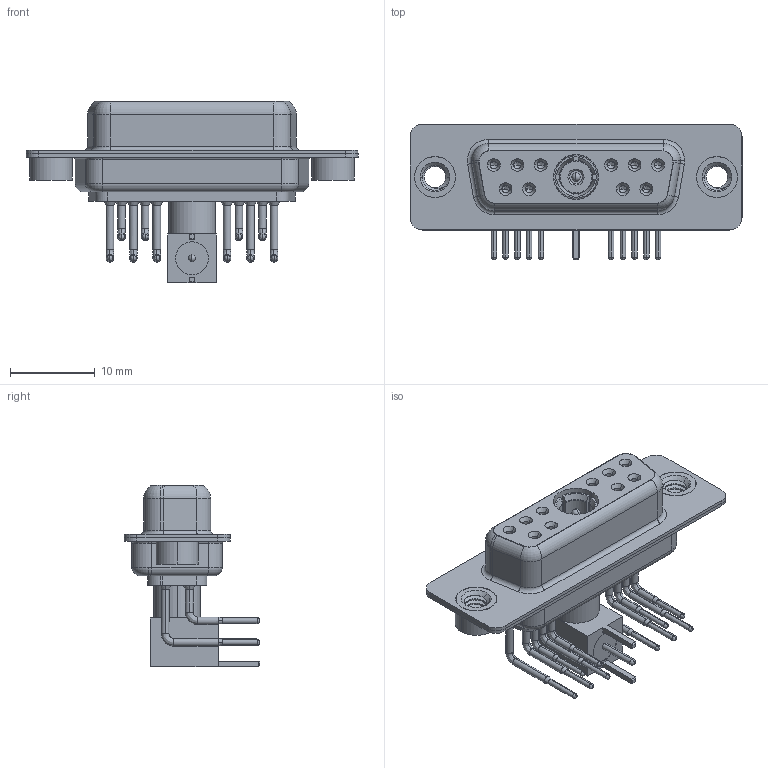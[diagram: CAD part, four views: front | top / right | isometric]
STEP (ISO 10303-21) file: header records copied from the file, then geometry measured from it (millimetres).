
FILE_DESCRIPTION (( 'STEP AP203' ), '1' );
FILE_NAME ('630-11W1640-7NA.STEP', '2022-05-31T14:39:56', ( '' ), ( '' ), 'SwSTEP 2.0', 'SolidWorks 2020', '' );
FILE_SCHEMA (( 'CONFIG_CONTROL_DESIGN' ));
Length unit declared in the file: millimetre
Products named in the file (14): 630Combo Threaded Rivet_A; 630Combo Contact Row 2; 630-11W1640-7NA; Insulator RA Pin; Locking Collar; 630Combo Shell Rear_15 Contacts; RA Back Shell; Co-Ax Plug_RA PC Tail; 630Combo Housing_11W1; 630Combo Contact Row 1; Pin_RA; Co-Ax Plug Assy_RA; Insulator Pin_Straight PC Tail; 630Combo Shell Front_15 Contacts
Assembly tree (22 placements, depth 3):
  630-11W1640-7NA
    630Combo Housing_11W1
    630Combo Shell Front_15 Contacts
    630Combo Shell Rear_15 Contacts
    630Combo Threaded Rivet_A  x2
    Co-Ax Plug Assy_RA
      Co-Ax Plug_RA PC Tail
      Insulator Pin_Straight PC Tail
      Pin_RA
      Locking Collar
      RA Back Shell
      Insulator RA Pin
    630Combo Contact Row 1  x6
    630Combo Contact Row 2  x4
Bounding box: 39.2 x 16 x 21.41 mm (x, y, z)
Volume: 2805.4 mm3; surface area: 6897 mm2
Topology: 21 solids, 21 shells, 971 faces, 2422 edges, 1520 vertices
Faces by surface type: cylinder 430, plane 284, cone 143, torus 63, bspline 47, sphere 4
Entity records: 21702 total; most frequent: CARTESIAN_POINT 5123, DIRECTION 3365, ORIENTED_EDGE 2944, EDGE_CURVE 1472, AXIS2_PLACEMENT_3D 1375, VERTEX_POINT 934, CIRCLE 740, EDGE_LOOP 724
